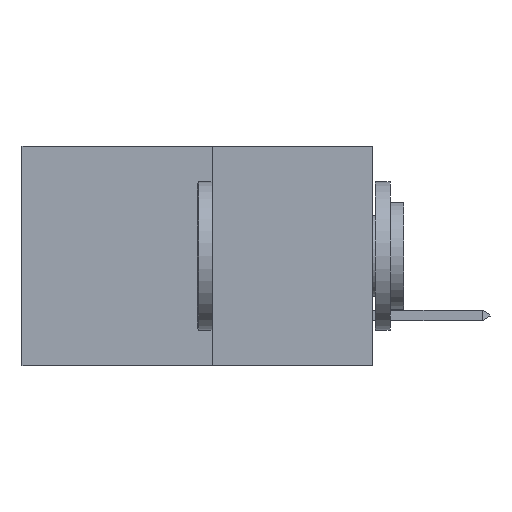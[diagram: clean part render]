
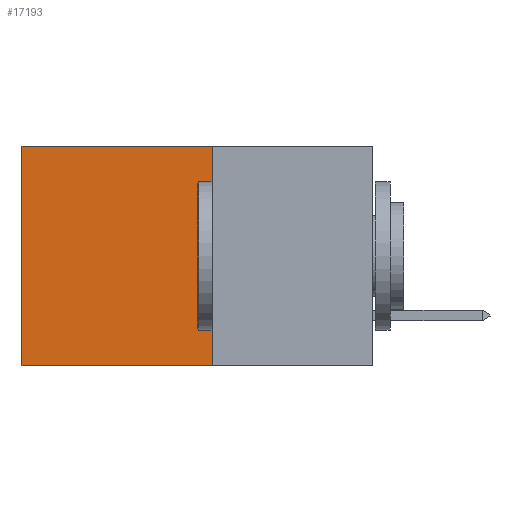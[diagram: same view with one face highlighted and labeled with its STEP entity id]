
A CAD part, left-side view. The second image highlights one B-rep face of the part: STEP entity #17193.
In plain terms, the highlighted planar face has unit normal (-1, 0, 0).
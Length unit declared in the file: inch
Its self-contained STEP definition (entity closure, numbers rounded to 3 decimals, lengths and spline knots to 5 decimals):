
#282 = DIRECTION ( 'NONE',  ( 0., 1., 0. ) ) ;
#617 = AXIS2_PLACEMENT_3D ( 'NONE', #15574, #12392, #2291 ) ;
#789 = CARTESIAN_POINT ( 'NONE',  ( 0.277, 0.27, 0. ) ) ;
#2131 = EDGE_LOOP ( 'NONE', ( #18409, #6235, #3532, #3387 ) ) ;
#2291 = DIRECTION ( 'NONE',  ( 0., 0., -1. ) ) ;
#2470 = EDGE_CURVE ( 'NONE', #18833, #14449, #7229, .T. ) ;
#3137 = CARTESIAN_POINT ( 'NONE',  ( 0.277, 0.27, -0.37 ) ) ;
#3387 = ORIENTED_EDGE ( 'NONE', *, *, #8460, .T. ) ;
#3532 = ORIENTED_EDGE ( 'NONE', *, *, #2470, .F. ) ;
#4740 = EDGE_CURVE ( 'NONE', #16760, #7964, #19118, .T. ) ;
#5205 = CARTESIAN_POINT ( 'NONE',  ( 0.277, 0.59, -0.37 ) ) ;
#5596 = DIRECTION ( 'NONE',  ( 0., 0., -1. ) ) ;
#6235 = ORIENTED_EDGE ( 'NONE', *, *, #14797, .F. ) ;
#6389 = CARTESIAN_POINT ( 'NONE',  ( 0.277, 0.59, 0. ) ) ;
#6560 = VECTOR ( 'NONE', #5596, 39.37008 ) ;
#7229 = LINE ( 'NONE', #17515, #15440 ) ;
#7964 = VERTEX_POINT ( 'NONE', #21295 ) ;
#8460 = EDGE_CURVE ( 'NONE', #18833, #16760, #19163, .T. ) ;
#8509 = VECTOR ( 'NONE', #13189, 39.37008 ) ;
#10786 = PLANE ( 'NONE',  #617 ) ;
#12392 = DIRECTION ( 'NONE',  ( 1., 0., 0. ) ) ;
#12416 = CARTESIAN_POINT ( 'NONE',  ( 0.277, 0.27, -0.37 ) ) ;
#13189 = DIRECTION ( 'NONE',  ( 0., 1., 0. ) ) ;
#14286 = FACE_OUTER_BOUND ( 'NONE', #2131, .T. ) ;
#14449 = VERTEX_POINT ( 'NONE', #12416 ) ;
#14797 = EDGE_CURVE ( 'NONE', #14449, #7964, #17720, .T. ) ;
#14851 = VECTOR ( 'NONE', #282, 39.37008 ) ;
#15440 = VECTOR ( 'NONE', #19023, 39.37008 ) ;
#15574 = CARTESIAN_POINT ( 'NONE',  ( 0.277, 0.27, -0.37 ) ) ;
#16760 = VERTEX_POINT ( 'NONE', #6389 ) ;
#17193 = ADVANCED_FACE ( 'NONE', ( #14286 ), #10786, .F. ) ;
#17515 = CARTESIAN_POINT ( 'NONE',  ( 0.277, 0.27, -0.37 ) ) ;
#17720 = LINE ( 'NONE', #3137, #8509 ) ;
#18409 = ORIENTED_EDGE ( 'NONE', *, *, #4740, .T. ) ;
#18833 = VERTEX_POINT ( 'NONE', #789 ) ;
#19023 = DIRECTION ( 'NONE',  ( 0., 0., -1. ) ) ;
#19118 = LINE ( 'NONE', #5205, #6560 ) ;
#19163 = LINE ( 'NONE', #20207, #14851 ) ;
#20207 = CARTESIAN_POINT ( 'NONE',  ( 0.277, 0.27, 0. ) ) ;
#21295 = CARTESIAN_POINT ( 'NONE',  ( 0.277, 0.59, -0.37 ) ) ;
